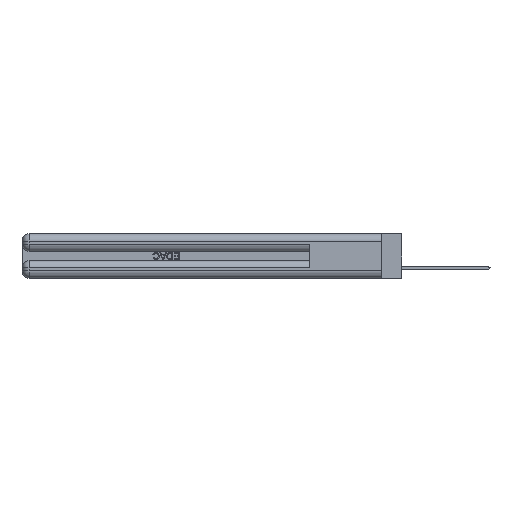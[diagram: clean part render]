
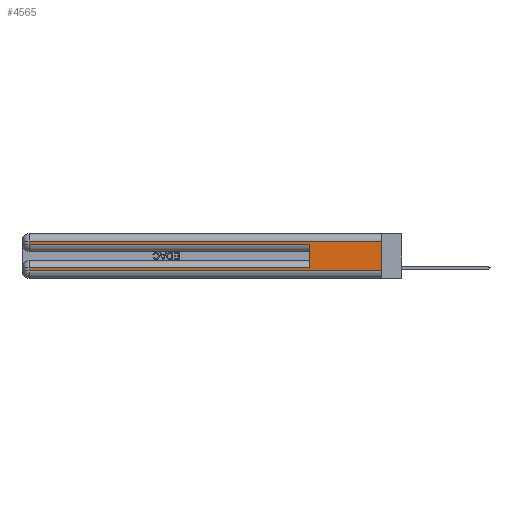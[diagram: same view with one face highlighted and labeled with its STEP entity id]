
A CAD part, left-side view. The second image highlights one B-rep face of the part: STEP entity #4565.
In plain terms, the highlighted planar face has unit normal (-1, 0, 0).
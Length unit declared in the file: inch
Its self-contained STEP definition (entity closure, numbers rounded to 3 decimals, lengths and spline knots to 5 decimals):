
#920 = DIRECTION ( 'NONE',  ( 0., 1., 0. ) ) ;
#1996 = LINE ( 'NONE', #33837, #48079 ) ;
#3265 = VECTOR ( 'NONE', #49454, 39.37008 ) ;
#4565 = ADVANCED_FACE ( 'NONE', ( #10878 ), #43766, .F. ) ;
#5054 = VERTEX_POINT ( 'NONE', #42892 ) ;
#5672 = CARTESIAN_POINT ( 'NONE',  ( 0., 0.6, 0.085 ) ) ;
#7598 = CARTESIAN_POINT ( 'NONE',  ( 0., 2.94, 0.37 ) ) ;
#7667 = CARTESIAN_POINT ( 'NONE',  ( 0., 2.94, 0.085 ) ) ;
#7794 = ORIENTED_EDGE ( 'NONE', *, *, #19705, .F. ) ;
#10447 = EDGE_CURVE ( 'NONE', #24064, #41264, #49625, .T. ) ;
#10597 = VECTOR ( 'NONE', #33637, 39.37008 ) ;
#10878 = FACE_OUTER_BOUND ( 'NONE', #47223, .T. ) ;
#11149 = LINE ( 'NONE', #35665, #24684 ) ;
#12178 = DIRECTION ( 'NONE',  ( 1., 0., 0. ) ) ;
#13160 = EDGE_CURVE ( 'NONE', #17150, #5054, #1996, .T. ) ;
#13428 = AXIS2_PLACEMENT_3D ( 'NONE', #35740, #12178, #20203 ) ;
#14162 = ORIENTED_EDGE ( 'NONE', *, *, #13160, .T. ) ;
#14390 = CARTESIAN_POINT ( 'NONE',  ( 0., 0., 0.06 ) ) ;
#16376 = VECTOR ( 'NONE', #23053, 39.37008 ) ;
#17150 = VERTEX_POINT ( 'NONE', #29098 ) ;
#17490 = ORIENTED_EDGE ( 'NONE', *, *, #29180, .T. ) ;
#18813 = CARTESIAN_POINT ( 'NONE',  ( 0., 0., 0.06 ) ) ;
#19705 = EDGE_CURVE ( 'NONE', #23733, #41917, #11149, .T. ) ;
#20026 = VECTOR ( 'NONE', #42836, 39.37008 ) ;
#20203 = DIRECTION ( 'NONE',  ( 0., 0., -1. ) ) ;
#23053 = DIRECTION ( 'NONE',  ( 0., -1., 0. ) ) ;
#23733 = VERTEX_POINT ( 'NONE', #5672 ) ;
#24064 = VERTEX_POINT ( 'NONE', #7667 ) ;
#24684 = VECTOR ( 'NONE', #47639, 39.37008 ) ;
#25515 = VECTOR ( 'NONE', #33677, 39.37008 ) ;
#25888 = CARTESIAN_POINT ( 'NONE',  ( 0., 0.6, 0.285 ) ) ;
#26802 = CARTESIAN_POINT ( 'NONE',  ( 0., 2.94, 0.285 ) ) ;
#29098 = CARTESIAN_POINT ( 'NONE',  ( 0., 0., 0.31 ) ) ;
#29180 = EDGE_CURVE ( 'NONE', #38610, #41917, #39795, .T. ) ;
#30282 = LINE ( 'NONE', #36937, #10597 ) ;
#30919 = CARTESIAN_POINT ( 'NONE',  ( 0., 2.94, 0.37 ) ) ;
#31196 = EDGE_CURVE ( 'NONE', #17150, #45674, #30282, .T. ) ;
#31442 = DIRECTION ( 'NONE',  ( 0., 0., -1. ) ) ;
#33637 = DIRECTION ( 'NONE',  ( 0., 0., -1. ) ) ;
#33677 = DIRECTION ( 'NONE',  ( 0., -1., 0. ) ) ;
#33837 = CARTESIAN_POINT ( 'NONE',  ( 0., 0., 0.31 ) ) ;
#33891 = ORIENTED_EDGE ( 'NONE', *, *, #10447, .T. ) ;
#34637 = LINE ( 'NONE', #41587, #3265 ) ;
#35137 = ORIENTED_EDGE ( 'NONE', *, *, #46267, .T. ) ;
#35609 = EDGE_CURVE ( 'NONE', #41264, #45674, #41560, .T. ) ;
#35665 = CARTESIAN_POINT ( 'NONE',  ( 0., 0.6, 0.145 ) ) ;
#35740 = CARTESIAN_POINT ( 'NONE',  ( 0., 0., 0.37 ) ) ;
#36937 = CARTESIAN_POINT ( 'NONE',  ( 0., 0., 0.37 ) ) ;
#38610 = VERTEX_POINT ( 'NONE', #26802 ) ;
#39795 = LINE ( 'NONE', #50075, #16376 ) ;
#41264 = VERTEX_POINT ( 'NONE', #42486 ) ;
#41560 = LINE ( 'NONE', #14390, #25515 ) ;
#41587 = CARTESIAN_POINT ( 'NONE',  ( 0., 0., 0.085 ) ) ;
#41681 = VECTOR ( 'NONE', #31442, 39.37008 ) ;
#41898 = EDGE_CURVE ( 'NONE', #23733, #24064, #34637, .T. ) ;
#41917 = VERTEX_POINT ( 'NONE', #25888 ) ;
#42486 = CARTESIAN_POINT ( 'NONE',  ( 0., 2.94, 0.06 ) ) ;
#42710 = ORIENTED_EDGE ( 'NONE', *, *, #35609, .T. ) ;
#42836 = DIRECTION ( 'NONE',  ( 0., 0., -1. ) ) ;
#42892 = CARTESIAN_POINT ( 'NONE',  ( 0., 2.94, 0.31 ) ) ;
#43458 = ORIENTED_EDGE ( 'NONE', *, *, #31196, .F. ) ;
#43766 = PLANE ( 'NONE',  #13428 ) ;
#44274 = ORIENTED_EDGE ( 'NONE', *, *, #41898, .T. ) ;
#44680 = LINE ( 'NONE', #7598, #20026 ) ;
#45674 = VERTEX_POINT ( 'NONE', #18813 ) ;
#46267 = EDGE_CURVE ( 'NONE', #5054, #38610, #44680, .T. ) ;
#47223 = EDGE_LOOP ( 'NONE', ( #43458, #14162, #35137, #17490, #7794, #44274, #33891, #42710 ) ) ;
#47639 = DIRECTION ( 'NONE',  ( 0., 0., 1. ) ) ;
#48079 = VECTOR ( 'NONE', #920, 39.37008 ) ;
#49454 = DIRECTION ( 'NONE',  ( 0., 1., 0. ) ) ;
#49625 = LINE ( 'NONE', #30919, #41681 ) ;
#50075 = CARTESIAN_POINT ( 'NONE',  ( 0., 0., 0.285 ) ) ;
